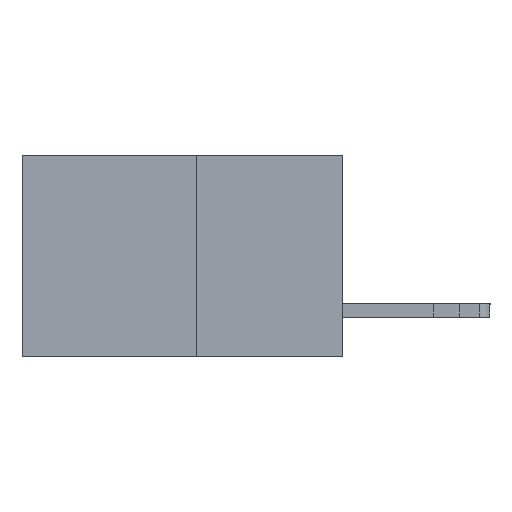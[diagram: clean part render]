
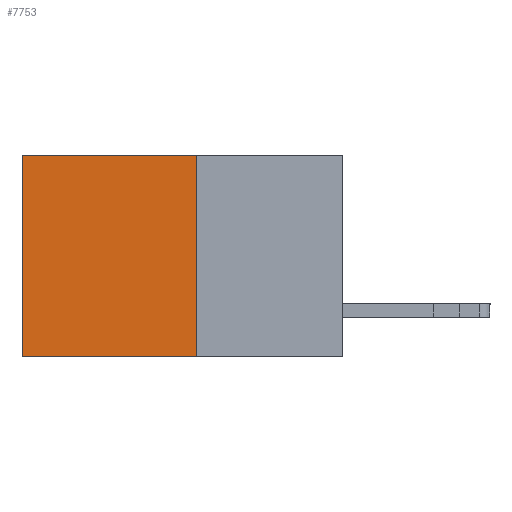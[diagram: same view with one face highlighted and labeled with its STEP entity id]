
A CAD part, left-side view. The second image highlights one B-rep face of the part: STEP entity #7753.
In plain terms, the highlighted planar face has unit normal (-1, 0, 0).
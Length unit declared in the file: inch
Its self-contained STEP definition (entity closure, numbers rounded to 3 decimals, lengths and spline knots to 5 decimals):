
#353 = EDGE_CURVE ( 'NONE', #21972, #5484, #1267, .T. ) ;
#694 = CARTESIAN_POINT ( 'NONE',  ( 0.277, 0.59, 0. ) ) ;
#1122 = CARTESIAN_POINT ( 'NONE',  ( 0.277, 0.27, -0.37 ) ) ;
#1264 = LINE ( 'NONE', #17063, #1895 ) ;
#1267 = LINE ( 'NONE', #1588, #21011 ) ;
#1588 = CARTESIAN_POINT ( 'NONE',  ( 0.277, 0.59, -0.37 ) ) ;
#1820 = LINE ( 'NONE', #15677, #2425 ) ;
#1895 = VECTOR ( 'NONE', #17144, 39.37008 ) ;
#2425 = VECTOR ( 'NONE', #11755, 39.37008 ) ;
#3038 = DIRECTION ( 'NONE',  ( 0., 0., -1. ) ) ;
#3549 = CARTESIAN_POINT ( 'NONE',  ( 0.277, 0.27, -0.37 ) ) ;
#4315 = EDGE_LOOP ( 'NONE', ( #7326, #13591, #22879, #9506 ) ) ;
#4974 = CARTESIAN_POINT ( 'NONE',  ( 0.277, 0.27, 0. ) ) ;
#5484 = VERTEX_POINT ( 'NONE', #14792 ) ;
#7326 = ORIENTED_EDGE ( 'NONE', *, *, #353, .T. ) ;
#7753 = ADVANCED_FACE ( 'NONE', ( #19506 ), #10171, .F. ) ;
#8989 = VECTOR ( 'NONE', #12629, 39.37008 ) ;
#9241 = VERTEX_POINT ( 'NONE', #4974 ) ;
#9397 = VERTEX_POINT ( 'NONE', #3549 ) ;
#9506 = ORIENTED_EDGE ( 'NONE', *, *, #22371, .T. ) ;
#9588 = LINE ( 'NONE', #1122, #8989 ) ;
#9913 = EDGE_CURVE ( 'NONE', #9241, #9397, #9588, .T. ) ;
#10171 = PLANE ( 'NONE',  #23730 ) ;
#11755 = DIRECTION ( 'NONE',  ( 0., 1., 0. ) ) ;
#12107 = DIRECTION ( 'NONE',  ( 0., 0., -1. ) ) ;
#12629 = DIRECTION ( 'NONE',  ( 0., 0., -1. ) ) ;
#13591 = ORIENTED_EDGE ( 'NONE', *, *, #15250, .F. ) ;
#14792 = CARTESIAN_POINT ( 'NONE',  ( 0.277, 0.59, -0.37 ) ) ;
#15250 = EDGE_CURVE ( 'NONE', #9397, #5484, #1820, .T. ) ;
#15677 = CARTESIAN_POINT ( 'NONE',  ( 0.277, 0.27, -0.37 ) ) ;
#17063 = CARTESIAN_POINT ( 'NONE',  ( 0.277, 0.27, 0. ) ) ;
#17144 = DIRECTION ( 'NONE',  ( 0., 1., 0. ) ) ;
#17782 = CARTESIAN_POINT ( 'NONE',  ( 0.277, 0.27, -0.37 ) ) ;
#19506 = FACE_OUTER_BOUND ( 'NONE', #4315, .T. ) ;
#21011 = VECTOR ( 'NONE', #3038, 39.37008 ) ;
#21972 = VERTEX_POINT ( 'NONE', #694 ) ;
#22371 = EDGE_CURVE ( 'NONE', #9241, #21972, #1264, .T. ) ;
#22879 = ORIENTED_EDGE ( 'NONE', *, *, #9913, .F. ) ;
#23458 = DIRECTION ( 'NONE',  ( 1., 0., 0. ) ) ;
#23730 = AXIS2_PLACEMENT_3D ( 'NONE', #17782, #23458, #12107 ) ;
